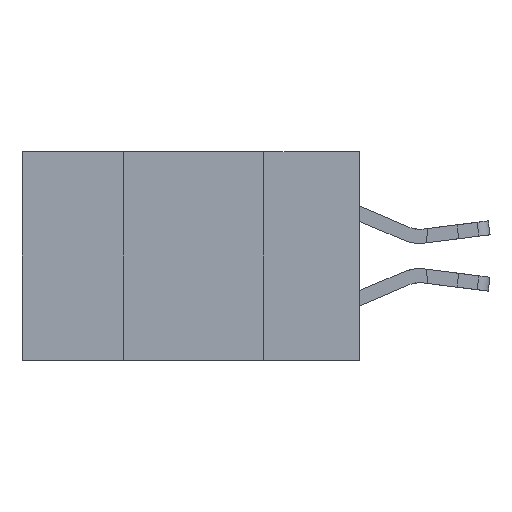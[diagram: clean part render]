
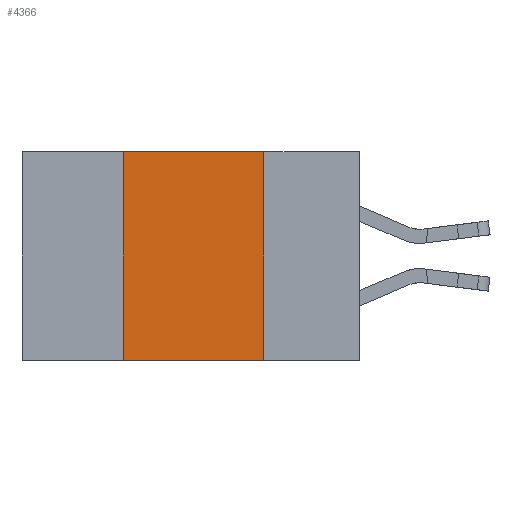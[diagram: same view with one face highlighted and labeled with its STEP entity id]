
A CAD part, left-side view. The second image highlights one B-rep face of the part: STEP entity #4366.
In plain terms, the highlighted planar face has unit normal (-1, 0, 0).
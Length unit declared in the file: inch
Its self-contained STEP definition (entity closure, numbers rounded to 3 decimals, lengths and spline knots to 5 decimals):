
#105 = EDGE_LOOP ( 'NONE', ( #26221, #7457, #26842, #20475 ) ) ;
#523 = EDGE_CURVE ( 'NONE', #26096, #26199, #9106, .T. ) ;
#593 = DIRECTION ( 'NONE',  ( 0., 0., -1. ) ) ;
#734 = AXIS2_PLACEMENT_3D ( 'NONE', #26405, #9533, #593 ) ;
#2205 = CARTESIAN_POINT ( 'NONE',  ( 0., 0.17, -0.37 ) ) ;
#3066 = CARTESIAN_POINT ( 'NONE',  ( 0., 0.17, 0. ) ) ;
#3159 = CARTESIAN_POINT ( 'NONE',  ( 0., 0.17, 0. ) ) ;
#4366 = ADVANCED_FACE ( 'NONE', ( #20575 ), #26548, .F. ) ;
#5002 = CARTESIAN_POINT ( 'NONE',  ( 0., 0.6, 0. ) ) ;
#5380 = EDGE_CURVE ( 'NONE', #27609, #18008, #22626, .T. ) ;
#7457 = ORIENTED_EDGE ( 'NONE', *, *, #523, .F. ) ;
#7603 = LINE ( 'NONE', #3066, #13591 ) ;
#8200 = CARTESIAN_POINT ( 'NONE',  ( 0., 0.42, 0. ) ) ;
#8788 = EDGE_CURVE ( 'NONE', #27609, #26096, #10163, .T. ) ;
#9106 = LINE ( 'NONE', #5002, #16460 ) ;
#9533 = DIRECTION ( 'NONE',  ( 1., 0., 0. ) ) ;
#10163 = LINE ( 'NONE', #8200, #19605 ) ;
#10166 = VECTOR ( 'NONE', #22906, 39.37008 ) ;
#10432 = EDGE_CURVE ( 'NONE', #26199, #18008, #7603, .T. ) ;
#11490 = DIRECTION ( 'NONE',  ( 0., -1., 0. ) ) ;
#12165 = CARTESIAN_POINT ( 'NONE',  ( 0., 0.42, -0.37 ) ) ;
#13337 = CARTESIAN_POINT ( 'NONE',  ( 0., 0.42, 0. ) ) ;
#13591 = VECTOR ( 'NONE', #20340, 39.37008 ) ;
#16460 = VECTOR ( 'NONE', #11490, 39.37008 ) ;
#17081 = DIRECTION ( 'NONE',  ( 0., 0., 1. ) ) ;
#18008 = VERTEX_POINT ( 'NONE', #2205 ) ;
#19605 = VECTOR ( 'NONE', #17081, 39.37008 ) ;
#20340 = DIRECTION ( 'NONE',  ( 0., 0., -1. ) ) ;
#20475 = ORIENTED_EDGE ( 'NONE', *, *, #5380, .T. ) ;
#20575 = FACE_OUTER_BOUND ( 'NONE', #105, .T. ) ;
#22626 = LINE ( 'NONE', #25186, #10166 ) ;
#22906 = DIRECTION ( 'NONE',  ( 0., -1., 0. ) ) ;
#25186 = CARTESIAN_POINT ( 'NONE',  ( 0., 0.6, -0.37 ) ) ;
#26096 = VERTEX_POINT ( 'NONE', #13337 ) ;
#26199 = VERTEX_POINT ( 'NONE', #3159 ) ;
#26221 = ORIENTED_EDGE ( 'NONE', *, *, #10432, .F. ) ;
#26405 = CARTESIAN_POINT ( 'NONE',  ( 0., 0.6, 0. ) ) ;
#26548 = PLANE ( 'NONE',  #734 ) ;
#26842 = ORIENTED_EDGE ( 'NONE', *, *, #8788, .F. ) ;
#27609 = VERTEX_POINT ( 'NONE', #12165 ) ;
